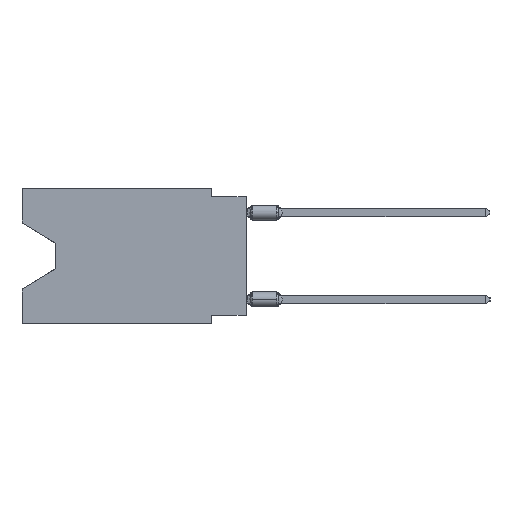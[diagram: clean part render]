
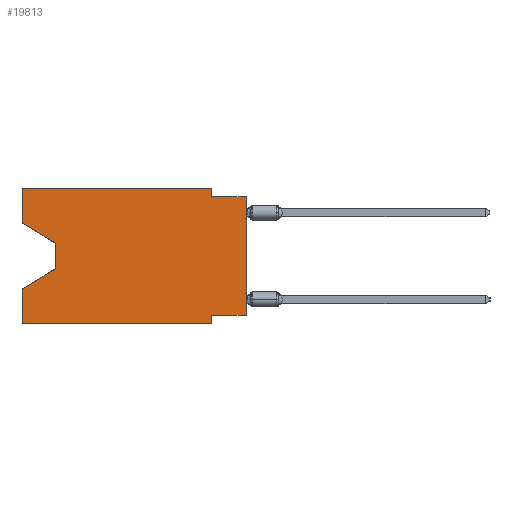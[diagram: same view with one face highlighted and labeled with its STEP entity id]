
A CAD part, left-side view. The second image highlights one B-rep face of the part: STEP entity #19813.
In plain terms, the highlighted planar face has unit normal (-1, 0, 0).
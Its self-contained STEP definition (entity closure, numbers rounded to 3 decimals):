
#596 = EDGE_CURVE ( 'NONE', #33176, #10933, #8467, .T. ) ;
#643 = ORIENTED_EDGE ( 'NONE', *, *, #23414, .T. ) ;
#649 = VECTOR ( 'NONE', #13995, 1000. ) ;
#718 = EDGE_CURVE ( 'NONE', #29742, #9208, #5522, .T. ) ;
#1073 = DIRECTION ( 'NONE',  ( 0., 0., -1. ) ) ;
#1139 = ORIENTED_EDGE ( 'NONE', *, *, #596, .T. ) ;
#1567 = CARTESIAN_POINT ( 'NONE',  ( 0., 16.383, -9.906 ) ) ;
#2224 = CARTESIAN_POINT ( 'NONE',  ( 0., 0., -9.271 ) ) ;
#2858 = CARTESIAN_POINT ( 'NONE',  ( 0., 0., -0.635 ) ) ;
#3837 = VERTEX_POINT ( 'NONE', #33171 ) ;
#4597 = EDGE_CURVE ( 'NONE', #12619, #16475, #14203, .T. ) ;
#4868 = CARTESIAN_POINT ( 'NONE',  ( 0., 16.383, 0. ) ) ;
#5104 = DIRECTION ( 'NONE',  ( 0., 0., -1. ) ) ;
#5142 = CARTESIAN_POINT ( 'NONE',  ( 0., 13.97, -4.013 ) ) ;
#5522 = LINE ( 'NONE', #10500, #5840 ) ;
#5840 = VECTOR ( 'NONE', #7759, 1000. ) ;
#6166 = CARTESIAN_POINT ( 'NONE',  ( 0., 16.383, -9.906 ) ) ;
#6743 = VERTEX_POINT ( 'NONE', #2858 ) ;
#7200 = VERTEX_POINT ( 'NONE', #1567 ) ;
#7524 = EDGE_CURVE ( 'NONE', #7200, #16475, #8581, .T. ) ;
#7543 = EDGE_CURVE ( 'NONE', #27031, #6743, #19083, .T. ) ;
#7704 = EDGE_CURVE ( 'NONE', #15015, #33176, #27334, .T. ) ;
#7759 = DIRECTION ( 'NONE',  ( 0., -1., 0. ) ) ;
#7991 = EDGE_CURVE ( 'NONE', #33155, #12619, #26785, .T. ) ;
#8083 = CARTESIAN_POINT ( 'NONE',  ( 0., 2.54, -0.635 ) ) ;
#8467 = LINE ( 'NONE', #14146, #22314 ) ;
#8581 = LINE ( 'NONE', #6166, #14117 ) ;
#8880 = CARTESIAN_POINT ( 'NONE',  ( 0., 0., -9.271 ) ) ;
#9192 = ORIENTED_EDGE ( 'NONE', *, *, #718, .F. ) ;
#9208 = VERTEX_POINT ( 'NONE', #10216 ) ;
#9645 = AXIS2_PLACEMENT_3D ( 'NONE', #25490, #17587, #28425 ) ;
#10016 = LINE ( 'NONE', #4868, #31551 ) ;
#10216 = CARTESIAN_POINT ( 'NONE',  ( 0., 2.54, 0. ) ) ;
#10375 = ORIENTED_EDGE ( 'NONE', *, *, #12886, .T. ) ;
#10500 = CARTESIAN_POINT ( 'NONE',  ( 0., 16.383, 0. ) ) ;
#10933 = VERTEX_POINT ( 'NONE', #17386 ) ;
#10995 = CARTESIAN_POINT ( 'NONE',  ( 0., 2.54, -9.271 ) ) ;
#12603 = DIRECTION ( 'NONE',  ( 0., 0., 1. ) ) ;
#12619 = VERTEX_POINT ( 'NONE', #10995 ) ;
#12886 = EDGE_CURVE ( 'NONE', #33155, #6743, #15117, .T. ) ;
#13571 = DIRECTION ( 'NONE',  ( 0., -1., 0. ) ) ;
#13995 = DIRECTION ( 'NONE',  ( 0., 0.855, -0.519 ) ) ;
#14117 = VECTOR ( 'NONE', #21483, 1000. ) ;
#14146 = CARTESIAN_POINT ( 'NONE',  ( 0., 13.97, -4.013 ) ) ;
#14203 = LINE ( 'NONE', #21602, #23827 ) ;
#14570 = ORIENTED_EDGE ( 'NONE', *, *, #30750, .F. ) ;
#14573 = ORIENTED_EDGE ( 'NONE', *, *, #7524, .T. ) ;
#15015 = VERTEX_POINT ( 'NONE', #31915 ) ;
#15037 = CARTESIAN_POINT ( 'NONE',  ( 0., 16.383, 0. ) ) ;
#15117 = LINE ( 'NONE', #33521, #16235 ) ;
#16235 = VECTOR ( 'NONE', #25774, 1000. ) ;
#16475 = VERTEX_POINT ( 'NONE', #28377 ) ;
#17386 = CARTESIAN_POINT ( 'NONE',  ( 0., 13.97, -5.893 ) ) ;
#17587 = DIRECTION ( 'NONE',  ( 1., 0., 0. ) ) ;
#18471 = EDGE_CURVE ( 'NONE', #15015, #29742, #10016, .T. ) ;
#18523 = VECTOR ( 'NONE', #13571, 1000. ) ;
#18764 = ORIENTED_EDGE ( 'NONE', *, *, #7704, .T. ) ;
#18975 = ORIENTED_EDGE ( 'NONE', *, *, #4597, .F. ) ;
#19008 = ORIENTED_EDGE ( 'NONE', *, *, #7543, .F. ) ;
#19083 = LINE ( 'NONE', #32319, #18523 ) ;
#19087 = VECTOR ( 'NONE', #27848, 1000. ) ;
#19347 = ORIENTED_EDGE ( 'NONE', *, *, #7991, .F. ) ;
#19761 = CARTESIAN_POINT ( 'NONE',  ( 0., 16.383, -2.546 ) ) ;
#19813 = ADVANCED_FACE ( 'NONE', ( #28822 ), #30997, .F. ) ;
#21093 = CARTESIAN_POINT ( 'NONE',  ( 0., 2.54, 0. ) ) ;
#21483 = DIRECTION ( 'NONE',  ( 0., -1., 0. ) ) ;
#21575 = VECTOR ( 'NONE', #5104, 1000. ) ;
#21595 = LINE ( 'NONE', #32093, #30797 ) ;
#21602 = CARTESIAN_POINT ( 'NONE',  ( 0., 2.54, -9.906 ) ) ;
#21615 = EDGE_CURVE ( 'NONE', #9208, #27031, #29177, .T. ) ;
#21746 = LINE ( 'NONE', #27073, #649 ) ;
#22005 = EDGE_LOOP ( 'NONE', ( #18764, #1139, #643, #14570, #14573, #18975, #19347, #10375, #19008, #32723, #9192, #28713 ) ) ;
#22314 = VECTOR ( 'NONE', #1073, 1000. ) ;
#23414 = EDGE_CURVE ( 'NONE', #10933, #3837, #21746, .T. ) ;
#23827 = VECTOR ( 'NONE', #27109, 1000. ) ;
#25490 = CARTESIAN_POINT ( 'NONE',  ( 0., 16.383, 0. ) ) ;
#25774 = DIRECTION ( 'NONE',  ( 0., 0., 1. ) ) ;
#26785 = LINE ( 'NONE', #8880, #33907 ) ;
#27031 = VERTEX_POINT ( 'NONE', #8083 ) ;
#27073 = CARTESIAN_POINT ( 'NONE',  ( 0., 13.97, -5.893 ) ) ;
#27109 = DIRECTION ( 'NONE',  ( 0., 0., -1. ) ) ;
#27118 = DIRECTION ( 'NONE',  ( 0., 1., 0. ) ) ;
#27334 = LINE ( 'NONE', #19761, #19087 ) ;
#27848 = DIRECTION ( 'NONE',  ( 0., -0.855, -0.519 ) ) ;
#28377 = CARTESIAN_POINT ( 'NONE',  ( 0., 2.54, -9.906 ) ) ;
#28425 = DIRECTION ( 'NONE',  ( 0., 0., -1. ) ) ;
#28713 = ORIENTED_EDGE ( 'NONE', *, *, #18471, .F. ) ;
#28822 = FACE_OUTER_BOUND ( 'NONE', #22005, .T. ) ;
#29177 = LINE ( 'NONE', #21093, #21575 ) ;
#29693 = DIRECTION ( 'NONE',  ( 0., 0., 1. ) ) ;
#29742 = VERTEX_POINT ( 'NONE', #15037 ) ;
#30750 = EDGE_CURVE ( 'NONE', #7200, #3837, #21595, .T. ) ;
#30797 = VECTOR ( 'NONE', #29693, 1000. ) ;
#30997 = PLANE ( 'NONE',  #9645 ) ;
#31551 = VECTOR ( 'NONE', #12603, 1000. ) ;
#31915 = CARTESIAN_POINT ( 'NONE',  ( 0., 16.383, -2.546 ) ) ;
#32093 = CARTESIAN_POINT ( 'NONE',  ( 0., 16.383, 0. ) ) ;
#32319 = CARTESIAN_POINT ( 'NONE',  ( 0., 0., -0.635 ) ) ;
#32723 = ORIENTED_EDGE ( 'NONE', *, *, #21615, .F. ) ;
#33155 = VERTEX_POINT ( 'NONE', #2224 ) ;
#33171 = CARTESIAN_POINT ( 'NONE',  ( 0., 16.383, -7.36 ) ) ;
#33176 = VERTEX_POINT ( 'NONE', #5142 ) ;
#33521 = CARTESIAN_POINT ( 'NONE',  ( 0., 0., 0. ) ) ;
#33907 = VECTOR ( 'NONE', #27118, 1000. ) ;
